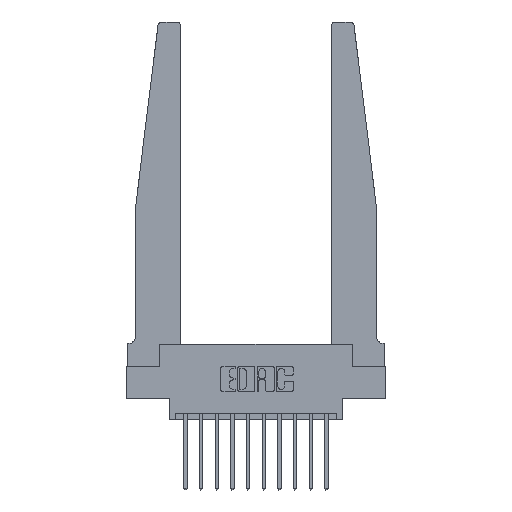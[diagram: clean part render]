
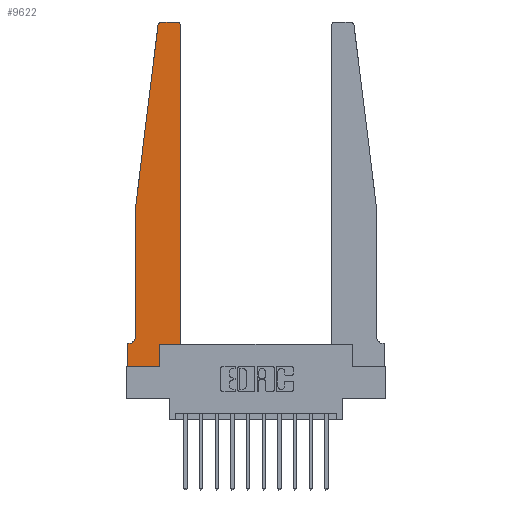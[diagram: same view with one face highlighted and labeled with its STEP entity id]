
A CAD part, top view. The second image highlights one B-rep face of the part: STEP entity #9622.
In plain terms, the highlighted planar face has unit normal (0, 0, 1).
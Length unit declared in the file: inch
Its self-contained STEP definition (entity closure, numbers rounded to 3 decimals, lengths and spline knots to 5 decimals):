
#29 = EDGE_CURVE ( 'NONE', #12580, #1513, #2586, .T. ) ;
#142 = DIRECTION ( 'NONE',  ( 0., 1., 0. ) ) ;
#256 = CARTESIAN_POINT ( 'NONE',  ( 0.065, 1.25, 0.37 ) ) ;
#395 = DIRECTION ( 'NONE',  ( 1., 0., 0. ) ) ;
#489 = DIRECTION ( 'NONE',  ( 1., 0., 0. ) ) ;
#569 = DIRECTION ( 'NONE',  ( 0., 0., 1. ) ) ;
#1045 = EDGE_CURVE ( 'NONE', #11328, #12580, #3648, .T. ) ;
#1278 = DIRECTION ( 'NONE',  ( -1., 0., 0. ) ) ;
#1436 = CARTESIAN_POINT ( 'NONE',  ( 0.2605, 0.18, 0.37 ) ) ;
#1513 = VERTEX_POINT ( 'NONE', #14779 ) ;
#1675 = ORIENTED_EDGE ( 'NONE', *, *, #14279, .T. ) ;
#1766 = ORIENTED_EDGE ( 'NONE', *, *, #8089, .T. ) ;
#1802 = VERTEX_POINT ( 'NONE', #4681 ) ;
#2058 = VECTOR ( 'NONE', #5292, 39.37008 ) ;
#2381 = CARTESIAN_POINT ( 'NONE',  ( 0.065, 1.25, 0.37 ) ) ;
#2536 = CARTESIAN_POINT ( 'NONE',  ( 0.425, 0.18, 0.37 ) ) ;
#2559 = CARTESIAN_POINT ( 'NONE',  ( 0.425, 2.72, 0.37 ) ) ;
#2586 = CIRCLE ( 'NONE', #3632, 0.05 ) ;
#2662 = LINE ( 'NONE', #1436, #4619 ) ;
#3017 = EDGE_CURVE ( 'NONE', #1513, #1802, #7655, .T. ) ;
#3041 = VECTOR ( 'NONE', #3719, 39.37008 ) ;
#3214 = DIRECTION ( 'NONE',  ( 1., 0., 0. ) ) ;
#3632 = AXIS2_PLACEMENT_3D ( 'NONE', #14841, #13126, #9262 ) ;
#3639 = LINE ( 'NONE', #12559, #3041 ) ;
#3648 = LINE ( 'NONE', #13796, #15977 ) ;
#3650 = CARTESIAN_POINT ( 'NONE',  ( 0.25, 2.75, 0.37 ) ) ;
#3719 = DIRECTION ( 'NONE',  ( 1., 0., 0. ) ) ;
#3853 = EDGE_CURVE ( 'NONE', #8924, #13919, #12765, .T. ) ;
#4157 = ORIENTED_EDGE ( 'NONE', *, *, #8763, .T. ) ;
#4203 = CARTESIAN_POINT ( 'NONE',  ( 0.425, 0.18, 0.37 ) ) ;
#4619 = VECTOR ( 'NONE', #142, 39.37008 ) ;
#4681 = CARTESIAN_POINT ( 'NONE',  ( 0., 0.1875, 0.37 ) ) ;
#4764 = VECTOR ( 'NONE', #12530, 39.37008 ) ;
#4814 = CARTESIAN_POINT ( 'NONE',  ( 0.395, 2.75, 0.37 ) ) ;
#5292 = DIRECTION ( 'NONE',  ( 0., -1., 0. ) ) ;
#5417 = ORIENTED_EDGE ( 'NONE', *, *, #6881, .T. ) ;
#5506 = VERTEX_POINT ( 'NONE', #14211 ) ;
#5508 = ORIENTED_EDGE ( 'NONE', *, *, #3853, .T. ) ;
#5627 = AXIS2_PLACEMENT_3D ( 'NONE', #6439, #569, #489 ) ;
#5892 = AXIS2_PLACEMENT_3D ( 'NONE', #9439, #14431, #3214 ) ;
#6439 = CARTESIAN_POINT ( 'NONE',  ( 0.27653, 2.72, 0.37 ) ) ;
#6465 = VECTOR ( 'NONE', #11445, 39.37008 ) ;
#6881 = EDGE_CURVE ( 'NONE', #10268, #11328, #14220, .T. ) ;
#7655 = LINE ( 'NONE', #11421, #10746 ) ;
#7848 = LINE ( 'NONE', #13086, #2058 ) ;
#8038 = CARTESIAN_POINT ( 'NONE',  ( 0.2605, 0., 0.37 ) ) ;
#8089 = EDGE_CURVE ( 'NONE', #1802, #5506, #7848, .T. ) ;
#8276 = EDGE_CURVE ( 'NONE', #14956, #12287, #2662, .T. ) ;
#8715 = CARTESIAN_POINT ( 'NONE',  ( 0., 0., 0.37 ) ) ;
#8763 = EDGE_CURVE ( 'NONE', #12287, #8924, #3639, .T. ) ;
#8781 = VECTOR ( 'NONE', #13788, 39.37008 ) ;
#8924 = VERTEX_POINT ( 'NONE', #4203 ) ;
#9204 = ORIENTED_EDGE ( 'NONE', *, *, #13438, .T. ) ;
#9206 = FACE_OUTER_BOUND ( 'NONE', #11620, .T. ) ;
#9262 = DIRECTION ( 'NONE',  ( -1., 0., 0. ) ) ;
#9439 = CARTESIAN_POINT ( 'NONE',  ( 0.395, 2.72, 0.37 ) ) ;
#9622 = ADVANCED_FACE ( 'NONE', ( #9206 ), #14135, .T. ) ;
#9817 = CARTESIAN_POINT ( 'NONE',  ( 0.065, 0.2375, 0.37 ) ) ;
#9866 = DIRECTION ( 'NONE',  ( 0., -1., 0. ) ) ;
#10123 = ORIENTED_EDGE ( 'NONE', *, *, #13828, .T. ) ;
#10268 = VERTEX_POINT ( 'NONE', #13220 ) ;
#10590 = CIRCLE ( 'NONE', #5892, 0.03 ) ;
#10746 = VECTOR ( 'NONE', #11107, 39.37008 ) ;
#11107 = DIRECTION ( 'NONE',  ( -1., 0., 0. ) ) ;
#11328 = VERTEX_POINT ( 'NONE', #2381 ) ;
#11386 = CARTESIAN_POINT ( 'NONE',  ( 0.2605, 0.18, 0.37 ) ) ;
#11421 = CARTESIAN_POINT ( 'NONE',  ( 0.065, 0.1875, 0.37 ) ) ;
#11445 = DIRECTION ( 'NONE',  ( -0.122, -0.992, 0. ) ) ;
#11528 = ORIENTED_EDGE ( 'NONE', *, *, #29, .T. ) ;
#11620 = EDGE_LOOP ( 'NONE', ( #14208, #1675, #5417, #15375, #11528, #13713, #1766, #9204, #13519, #4157, #5508, #10123 ) ) ;
#12287 = VERTEX_POINT ( 'NONE', #11386 ) ;
#12530 = DIRECTION ( 'NONE',  ( 0., 1., 0. ) ) ;
#12559 = CARTESIAN_POINT ( 'NONE',  ( 0.425, 0.18, 0.37 ) ) ;
#12580 = VERTEX_POINT ( 'NONE', #9817 ) ;
#12685 = CIRCLE ( 'NONE', #5627, 0.03 ) ;
#12765 = LINE ( 'NONE', #2536, #4764 ) ;
#12905 = DIRECTION ( 'NONE',  ( 0., 0., 1. ) ) ;
#13086 = CARTESIAN_POINT ( 'NONE',  ( 0., 0., 0.37 ) ) ;
#13126 = DIRECTION ( 'NONE',  ( 0., 0., -1. ) ) ;
#13220 = CARTESIAN_POINT ( 'NONE',  ( 0.24675, 2.72367, 0.37 ) ) ;
#13438 = EDGE_CURVE ( 'NONE', #5506, #14956, #14953, .T. ) ;
#13509 = CARTESIAN_POINT ( 'NONE',  ( 0.27653, 2.75, 0.37 ) ) ;
#13519 = ORIENTED_EDGE ( 'NONE', *, *, #8276, .T. ) ;
#13633 = LINE ( 'NONE', #3650, #16104 ) ;
#13713 = ORIENTED_EDGE ( 'NONE', *, *, #3017, .T. ) ;
#13788 = DIRECTION ( 'NONE',  ( 1., 0., 0. ) ) ;
#13796 = CARTESIAN_POINT ( 'NONE',  ( 0.065, 1.25, 0.37 ) ) ;
#13828 = EDGE_CURVE ( 'NONE', #13919, #15444, #10590, .T. ) ;
#13919 = VERTEX_POINT ( 'NONE', #2559 ) ;
#14026 = VERTEX_POINT ( 'NONE', #13509 ) ;
#14135 = PLANE ( 'NONE',  #16173 ) ;
#14208 = ORIENTED_EDGE ( 'NONE', *, *, #14529, .T. ) ;
#14211 = CARTESIAN_POINT ( 'NONE',  ( 0., 0., 0.37 ) ) ;
#14220 = LINE ( 'NONE', #256, #6465 ) ;
#14279 = EDGE_CURVE ( 'NONE', #14026, #10268, #12685, .T. ) ;
#14431 = DIRECTION ( 'NONE',  ( 0., 0., 1. ) ) ;
#14529 = EDGE_CURVE ( 'NONE', #15444, #14026, #13633, .T. ) ;
#14779 = CARTESIAN_POINT ( 'NONE',  ( 0.015, 0.1875, 0.37 ) ) ;
#14841 = CARTESIAN_POINT ( 'NONE',  ( 0.015, 0.2375, 0.37 ) ) ;
#14953 = LINE ( 'NONE', #8715, #8781 ) ;
#14956 = VERTEX_POINT ( 'NONE', #8038 ) ;
#15375 = ORIENTED_EDGE ( 'NONE', *, *, #1045, .T. ) ;
#15377 = CARTESIAN_POINT ( 'NONE',  ( 0., 0.1875, 0.37 ) ) ;
#15444 = VERTEX_POINT ( 'NONE', #4814 ) ;
#15977 = VECTOR ( 'NONE', #9866, 39.37008 ) ;
#16104 = VECTOR ( 'NONE', #1278, 39.37008 ) ;
#16173 = AXIS2_PLACEMENT_3D ( 'NONE', #15377, #12905, #395 ) ;
